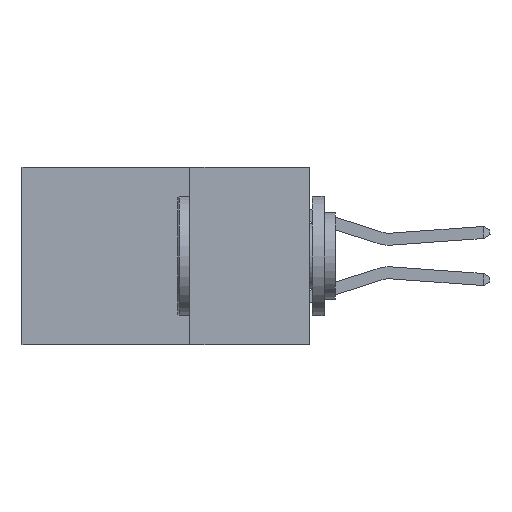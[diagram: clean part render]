
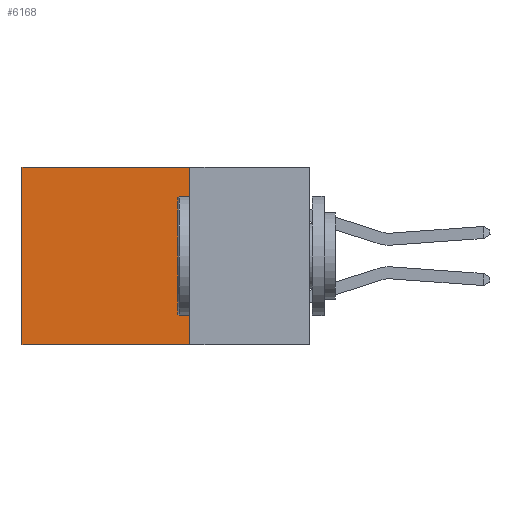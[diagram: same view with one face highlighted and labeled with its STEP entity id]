
A CAD part, left-side view. The second image highlights one B-rep face of the part: STEP entity #6168.
In plain terms, the highlighted planar face has unit normal (-1, 0, 0).
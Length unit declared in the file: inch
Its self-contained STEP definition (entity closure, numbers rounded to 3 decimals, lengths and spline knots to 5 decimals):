
#256 = AXIS2_PLACEMENT_3D ( 'NONE', #18234, #2040, #12547 ) ;
#801 = CARTESIAN_POINT ( 'NONE',  ( 0.2615, 0.6, -0.37 ) ) ;
#842 = ORIENTED_EDGE ( 'NONE', *, *, #18362, .T. ) ;
#2040 = DIRECTION ( 'NONE',  ( 1., 0., 0. ) ) ;
#4265 = DIRECTION ( 'NONE',  ( 0., 0., -1. ) ) ;
#5702 = DIRECTION ( 'NONE',  ( 0., 1., 0. ) ) ;
#6168 = ADVANCED_FACE ( 'NONE', ( #16879 ), #12365, .F. ) ;
#6224 = LINE ( 'NONE', #13657, #15903 ) ;
#6958 = CARTESIAN_POINT ( 'NONE',  ( 0.2615, 0.6, 0. ) ) ;
#7241 = CARTESIAN_POINT ( 'NONE',  ( 0.2615, 0.25, -0.37 ) ) ;
#7599 = VERTEX_POINT ( 'NONE', #16726 ) ;
#8600 = CARTESIAN_POINT ( 'NONE',  ( 0.2615, 0.25, -0.37 ) ) ;
#8988 = CARTESIAN_POINT ( 'NONE',  ( 0.2615, 0.25, 0. ) ) ;
#9495 = EDGE_CURVE ( 'NONE', #13503, #16921, #12741, .T. ) ;
#9586 = VERTEX_POINT ( 'NONE', #6958 ) ;
#9955 = ORIENTED_EDGE ( 'NONE', *, *, #11481, .T. ) ;
#10425 = LINE ( 'NONE', #8988, #10767 ) ;
#10767 = VECTOR ( 'NONE', #5702, 39.37008 ) ;
#11063 = VECTOR ( 'NONE', #15738, 39.37008 ) ;
#11211 = EDGE_LOOP ( 'NONE', ( #9955, #17222, #16512, #842 ) ) ;
#11481 = EDGE_CURVE ( 'NONE', #9586, #16921, #6224, .T. ) ;
#11674 = LINE ( 'NONE', #7241, #12459 ) ;
#12296 = DIRECTION ( 'NONE',  ( 0., 0., -1. ) ) ;
#12365 = PLANE ( 'NONE',  #256 ) ;
#12459 = VECTOR ( 'NONE', #4265, 39.37008 ) ;
#12547 = DIRECTION ( 'NONE',  ( 0., 0., -1. ) ) ;
#12741 = LINE ( 'NONE', #18814, #11063 ) ;
#13503 = VERTEX_POINT ( 'NONE', #8600 ) ;
#13616 = EDGE_CURVE ( 'NONE', #7599, #13503, #11674, .T. ) ;
#13657 = CARTESIAN_POINT ( 'NONE',  ( 0.2615, 0.6, -0.37 ) ) ;
#15738 = DIRECTION ( 'NONE',  ( 0., 1., 0. ) ) ;
#15903 = VECTOR ( 'NONE', #12296, 39.37008 ) ;
#16512 = ORIENTED_EDGE ( 'NONE', *, *, #13616, .F. ) ;
#16726 = CARTESIAN_POINT ( 'NONE',  ( 0.2615, 0.25, 0. ) ) ;
#16879 = FACE_OUTER_BOUND ( 'NONE', #11211, .T. ) ;
#16921 = VERTEX_POINT ( 'NONE', #801 ) ;
#17222 = ORIENTED_EDGE ( 'NONE', *, *, #9495, .F. ) ;
#18234 = CARTESIAN_POINT ( 'NONE',  ( 0.2615, 0.25, -0.37 ) ) ;
#18362 = EDGE_CURVE ( 'NONE', #7599, #9586, #10425, .T. ) ;
#18814 = CARTESIAN_POINT ( 'NONE',  ( 0.2615, 0.25, -0.37 ) ) ;
